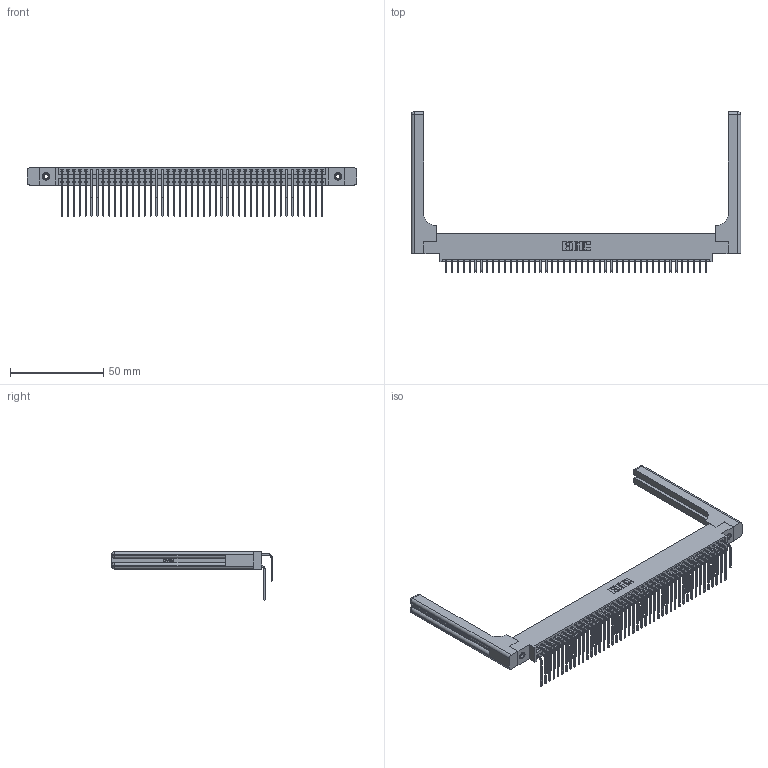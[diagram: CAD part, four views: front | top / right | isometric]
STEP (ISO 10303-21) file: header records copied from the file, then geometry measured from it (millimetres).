
FILE_DESCRIPTION (( 'STEP AP203' ), '1' );
FILE_NAME ('396-090-559-858.STEP', '2019-11-03T14:29:10', ( '' ), ( '' ), 'SwSTEP 2.0', 'SolidWorks 2016', '' );
FILE_SCHEMA (( 'CONFIG_CONTROL_DESIGN' ));
Length unit declared in the file: inch
Products named in the file (6): 346 Part_0.170 Offset - 0.156 Dia-TH; 345-250-001_345-250-001-102; 346-220-058_345-220-058; 345-292-001_558 559 Tail - 1; 396-090-559-858; 345-292-001_559 Tail - 2
Assembly tree (95 placements, depth 2):
  396-090-559-858
    346 Part_0.170 Offset - 0.156 Dia-TH
    345-292-001_558 559 Tail - 1  x45
    345-292-001_559 Tail - 2  x45
    345-250-001_345-250-001-102  x2
    346-220-058_345-220-058  x2
Bounding box: 176.94 x 86.17 x 26.16 mm (x, y, z)
Volume: 25135.6 mm3; surface area: 31939.5 mm2
Topology: 95 solids, 95 shells, 5242 faces, 15497 edges, 10190 vertices
Faces by surface type: plane 3558, cylinder 1624, bspline 36, cone 12, sphere 8, torus 4
Entity records: 36062 total; most frequent: CARTESIAN_POINT 7000, ORIENTED_EDGE 5680, DIRECTION 5124, EDGE_CURVE 2840, LINE 2396, VECTOR 2396, VERTEX_POINT 1882, AXIS2_PLACEMENT_3D 1364
